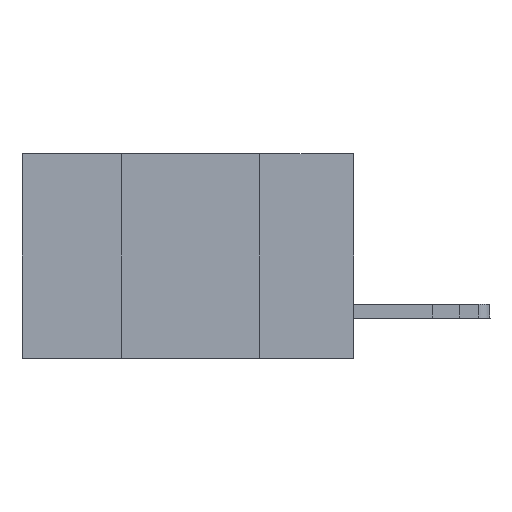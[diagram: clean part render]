
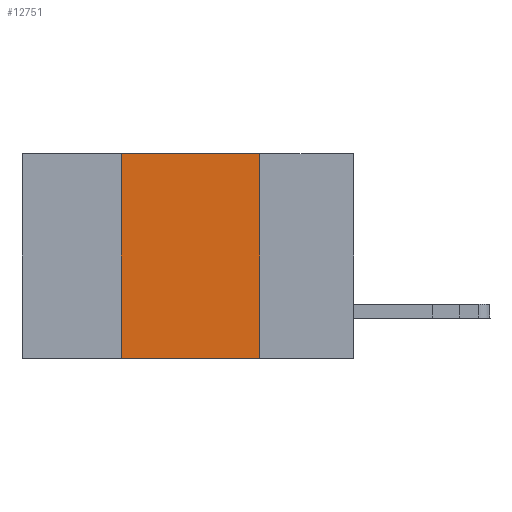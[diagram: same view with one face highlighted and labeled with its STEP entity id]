
A CAD part, left-side view. The second image highlights one B-rep face of the part: STEP entity #12751.
In plain terms, the highlighted planar face has unit normal (-1, 0, 0).
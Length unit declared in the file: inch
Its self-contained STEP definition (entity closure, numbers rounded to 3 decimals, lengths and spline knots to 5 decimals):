
#223 = EDGE_CURVE ( 'NONE', #19942, #4454, #1072, .T. ) ;
#328 = DIRECTION ( 'NONE',  ( 0., 0., -1. ) ) ;
#1072 = LINE ( 'NONE', #17238, #4771 ) ;
#1409 = VERTEX_POINT ( 'NONE', #21917 ) ;
#1745 = LINE ( 'NONE', #3526, #12907 ) ;
#1783 = DIRECTION ( 'NONE',  ( 0., -1., 0. ) ) ;
#2110 = CARTESIAN_POINT ( 'NONE',  ( 0., 0.6, 0. ) ) ;
#3526 = CARTESIAN_POINT ( 'NONE',  ( 0., 0.17, 0. ) ) ;
#4454 = VERTEX_POINT ( 'NONE', #22662 ) ;
#4771 = VECTOR ( 'NONE', #10048, 39.37008 ) ;
#6409 = EDGE_CURVE ( 'NONE', #9677, #19942, #11118, .T. ) ;
#6871 = CARTESIAN_POINT ( 'NONE',  ( 0., 0.42, 0. ) ) ;
#7146 = VECTOR ( 'NONE', #19990, 39.37008 ) ;
#8163 = EDGE_LOOP ( 'NONE', ( #21066, #13527, #20263, #10314 ) ) ;
#9311 = DIRECTION ( 'NONE',  ( 1., 0., 0. ) ) ;
#9677 = VERTEX_POINT ( 'NONE', #23550 ) ;
#10048 = DIRECTION ( 'NONE',  ( 0., -1., 0. ) ) ;
#10314 = ORIENTED_EDGE ( 'NONE', *, *, #14965, .T. ) ;
#11009 = CARTESIAN_POINT ( 'NONE',  ( 0., 0.42, 0. ) ) ;
#11118 = LINE ( 'NONE', #11009, #7146 ) ;
#12004 = CARTESIAN_POINT ( 'NONE',  ( 0., 0.6, -0.37 ) ) ;
#12408 = VECTOR ( 'NONE', #1783, 39.37008 ) ;
#12751 = ADVANCED_FACE ( 'NONE', ( #18533 ), #23560, .F. ) ;
#12907 = VECTOR ( 'NONE', #17689, 39.37008 ) ;
#13527 = ORIENTED_EDGE ( 'NONE', *, *, #223, .F. ) ;
#14965 = EDGE_CURVE ( 'NONE', #9677, #1409, #19305, .T. ) ;
#16529 = AXIS2_PLACEMENT_3D ( 'NONE', #2110, #9311, #328 ) ;
#17238 = CARTESIAN_POINT ( 'NONE',  ( 0., 0.6, 0. ) ) ;
#17689 = DIRECTION ( 'NONE',  ( 0., 0., -1. ) ) ;
#18533 = FACE_OUTER_BOUND ( 'NONE', #8163, .T. ) ;
#19305 = LINE ( 'NONE', #12004, #12408 ) ;
#19942 = VERTEX_POINT ( 'NONE', #6871 ) ;
#19990 = DIRECTION ( 'NONE',  ( 0., 0., 1. ) ) ;
#20263 = ORIENTED_EDGE ( 'NONE', *, *, #6409, .F. ) ;
#20757 = EDGE_CURVE ( 'NONE', #4454, #1409, #1745, .T. ) ;
#21066 = ORIENTED_EDGE ( 'NONE', *, *, #20757, .F. ) ;
#21917 = CARTESIAN_POINT ( 'NONE',  ( 0., 0.17, -0.37 ) ) ;
#22662 = CARTESIAN_POINT ( 'NONE',  ( 0., 0.17, 0. ) ) ;
#23550 = CARTESIAN_POINT ( 'NONE',  ( 0., 0.42, -0.37 ) ) ;
#23560 = PLANE ( 'NONE',  #16529 ) ;
